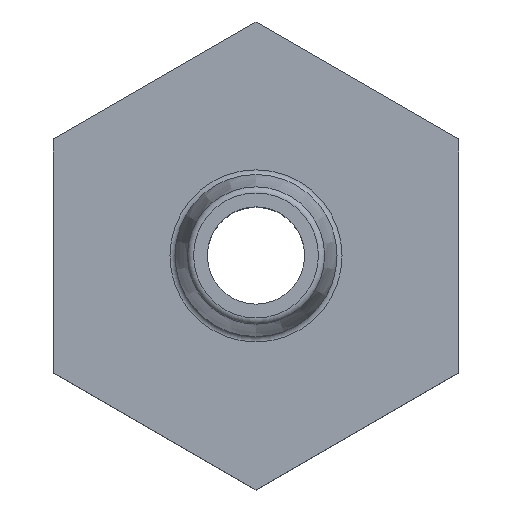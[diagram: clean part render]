
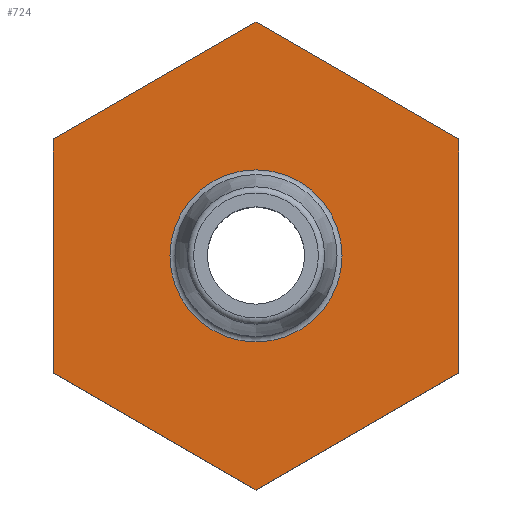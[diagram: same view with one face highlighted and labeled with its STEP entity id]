
A CAD part, top view. The second image highlights one B-rep face of the part: STEP entity #724.
In plain terms, the highlighted planar face has unit normal (0, 0, 1).
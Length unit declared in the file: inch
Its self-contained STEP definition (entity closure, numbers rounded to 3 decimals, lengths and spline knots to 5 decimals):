
#24=FACE_BOUND('',#120,.T.);
#31=PLANE('',#818);
#74=FACE_OUTER_BOUND('',#119,.T.);
#119=EDGE_LOOP('',(#641,#642,#643,#644,#645,#646));
#120=EDGE_LOOP('',(#647,#648));
#136=CIRCLE('',#773,0.23902);
#137=CIRCLE('',#774,0.23902);
#223=LINE('',#7310,#261);
#224=LINE('',#7312,#262);
#225=LINE('',#7314,#263);
#226=LINE('',#7316,#264);
#227=LINE('',#7318,#265);
#228=LINE('',#7319,#266);
#261=VECTOR('',#989,39.37008);
#262=VECTOR('',#990,39.37008);
#263=VECTOR('',#991,39.37008);
#264=VECTOR('',#992,39.37008);
#265=VECTOR('',#993,39.37008);
#266=VECTOR('',#994,39.37008);
#306=VERTEX_POINT('',#2909);
#307=VERTEX_POINT('',#2910);
#343=VERTEX_POINT('',#7308);
#344=VERTEX_POINT('',#7309);
#345=VERTEX_POINT('',#7311);
#346=VERTEX_POINT('',#7313);
#347=VERTEX_POINT('',#7315);
#348=VERTEX_POINT('',#7317);
#394=EDGE_CURVE('',#306,#307,#136,.T.);
#395=EDGE_CURVE('',#307,#306,#137,.T.);
#445=EDGE_CURVE('',#343,#344,#223,.T.);
#446=EDGE_CURVE('',#345,#343,#224,.T.);
#447=EDGE_CURVE('',#346,#345,#225,.T.);
#448=EDGE_CURVE('',#347,#346,#226,.T.);
#449=EDGE_CURVE('',#348,#347,#227,.T.);
#450=EDGE_CURVE('',#344,#348,#228,.T.);
#641=ORIENTED_EDGE('',*,*,#445,.F.);
#642=ORIENTED_EDGE('',*,*,#446,.F.);
#643=ORIENTED_EDGE('',*,*,#447,.F.);
#644=ORIENTED_EDGE('',*,*,#448,.F.);
#645=ORIENTED_EDGE('',*,*,#449,.F.);
#646=ORIENTED_EDGE('',*,*,#450,.F.);
#647=ORIENTED_EDGE('',*,*,#394,.T.);
#648=ORIENTED_EDGE('',*,*,#395,.T.);
#724=ADVANCED_FACE('',(#74,#24),#31,.F.);
#773=AXIS2_PLACEMENT_3D('',#2911,#883,#884);
#774=AXIS2_PLACEMENT_3D('',#2912,#885,#886);
#818=AXIS2_PLACEMENT_3D('',#7307,#987,#988);
#883=DIRECTION('center_axis',(0.,0.,-1.));
#884=DIRECTION('ref_axis',(-1.,0.,0.));
#885=DIRECTION('center_axis',(0.,0.,-1.));
#886=DIRECTION('ref_axis',(-1.,0.,0.));
#987=DIRECTION('center_axis',(0.,0.,-1.));
#988=DIRECTION('ref_axis',(-1.,0.,0.));
#989=DIRECTION('',(0.866,0.5,0.));
#990=DIRECTION('',(0.,1.,0.));
#991=DIRECTION('',(-0.866,0.5,0.));
#992=DIRECTION('',(-0.866,-0.5,0.));
#993=DIRECTION('',(0.,-1.,0.));
#994=DIRECTION('',(0.866,-0.5,0.));
#2909=CARTESIAN_POINT('',(-0.23902,0.,-0.17946));
#2910=CARTESIAN_POINT('',(0.23902,0.,-0.17946));
#2911=CARTESIAN_POINT('Origin',(0.,0.,
-0.17946));
#2912=CARTESIAN_POINT('Origin',(0.,0.,
-0.17946));
#7307=CARTESIAN_POINT('Origin',(0.,0.64952,-0.17946));
#7308=CARTESIAN_POINT('',(-0.5625,0.32476,-0.17946));
#7309=CARTESIAN_POINT('',(0.,0.64952,-0.17946));
#7310=CARTESIAN_POINT('',(-0.5625,0.32476,-0.17946));
#7311=CARTESIAN_POINT('',(-0.5625,-0.32476,-0.17946));
#7312=CARTESIAN_POINT('',(-0.5625,-0.32476,-0.17946));
#7313=CARTESIAN_POINT('',(0.,-0.64952,-0.17946));
#7314=CARTESIAN_POINT('',(0.,-0.64952,-0.17946));
#7315=CARTESIAN_POINT('',(0.5625,-0.32476,-0.17946));
#7316=CARTESIAN_POINT('',(0.5625,-0.32476,-0.17946));
#7317=CARTESIAN_POINT('',(0.5625,0.32476,-0.17946));
#7318=CARTESIAN_POINT('',(0.5625,0.32476,-0.17946));
#7319=CARTESIAN_POINT('',(0.,0.64952,-0.17946));
